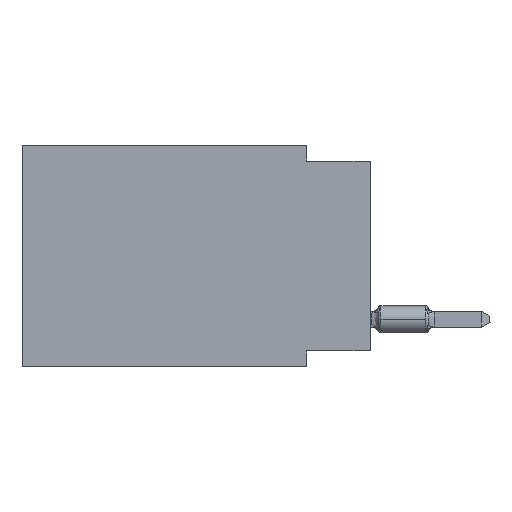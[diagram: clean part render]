
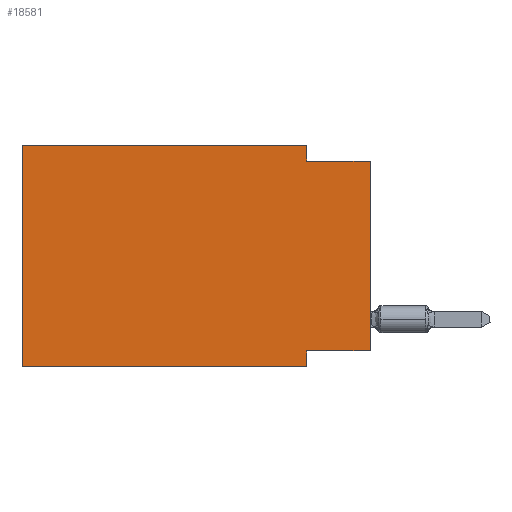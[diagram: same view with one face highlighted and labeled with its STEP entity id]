
A CAD part, left-side view. The second image highlights one B-rep face of the part: STEP entity #18581.
In plain terms, the highlighted planar face has unit normal (-1, 0, 0).
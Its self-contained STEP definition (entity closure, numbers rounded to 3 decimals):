
#150 = EDGE_CURVE ( 'NONE', #3956, #7314, #4441, .T. ) ;
#947 = ORIENTED_EDGE ( 'NONE', *, *, #33464, .F. ) ;
#1435 = DIRECTION ( 'NONE',  ( 0., 0., 1. ) ) ;
#3645 = DIRECTION ( 'NONE',  ( 0., -1., 0. ) ) ;
#3956 = VERTEX_POINT ( 'NONE', #19275 ) ;
#4171 = VERTEX_POINT ( 'NONE', #24043 ) ;
#4428 = ORIENTED_EDGE ( 'NONE', *, *, #22946, .F. ) ;
#4441 = LINE ( 'NONE', #12628, #32275 ) ;
#5887 = VECTOR ( 'NONE', #3645, 1000. ) ;
#6837 = ORIENTED_EDGE ( 'NONE', *, *, #17227, .F. ) ;
#7088 = FACE_OUTER_BOUND ( 'NONE', #22994, .T. ) ;
#7314 = VERTEX_POINT ( 'NONE', #27751 ) ;
#7979 = DIRECTION ( 'NONE',  ( 0., -1., 0. ) ) ;
#8051 = VECTOR ( 'NONE', #27856, 1000. ) ;
#9143 = CARTESIAN_POINT ( 'NONE',  ( 0., 0., -0.635 ) ) ;
#10374 = CARTESIAN_POINT ( 'NONE',  ( 0., 13.97, 0. ) ) ;
#10530 = ORIENTED_EDGE ( 'NONE', *, *, #19346, .F. ) ;
#10994 = VERTEX_POINT ( 'NONE', #25387 ) ;
#11420 = LINE ( 'NONE', #22230, #17637 ) ;
#11453 = VECTOR ( 'NONE', #1435, 1000. ) ;
#11707 = CARTESIAN_POINT ( 'NONE',  ( 0., 0., -8.255 ) ) ;
#11760 = CARTESIAN_POINT ( 'NONE',  ( 0., 13.97, 0. ) ) ;
#12628 = CARTESIAN_POINT ( 'NONE',  ( 0., 13.97, -8.89 ) ) ;
#13646 = VERTEX_POINT ( 'NONE', #28671 ) ;
#13700 = ORIENTED_EDGE ( 'NONE', *, *, #17064, .F. ) ;
#17064 = EDGE_CURVE ( 'NONE', #10994, #18953, #30346, .T. ) ;
#17227 = EDGE_CURVE ( 'NONE', #18953, #7314, #17358, .T. ) ;
#17240 = ORIENTED_EDGE ( 'NONE', *, *, #28916, .T. ) ;
#17358 = LINE ( 'NONE', #20036, #34678 ) ;
#17637 = VECTOR ( 'NONE', #27726, 1000. ) ;
#17889 = DIRECTION ( 'NONE',  ( 0., 0., -1. ) ) ;
#18253 = DIRECTION ( 'NONE',  ( 1., 0., 0. ) ) ;
#18581 = ADVANCED_FACE ( 'NONE', ( #7088 ), #23927, .F. ) ;
#18953 = VERTEX_POINT ( 'NONE', #22840 ) ;
#19275 = CARTESIAN_POINT ( 'NONE',  ( 0., 13.97, -8.89 ) ) ;
#19346 = EDGE_CURVE ( 'NONE', #20024, #4171, #19947, .T. ) ;
#19947 = LINE ( 'NONE', #9143, #5887 ) ;
#20024 = VERTEX_POINT ( 'NONE', #29822 ) ;
#20036 = CARTESIAN_POINT ( 'NONE',  ( 0., 2.54, -8.89 ) ) ;
#20688 = EDGE_CURVE ( 'NONE', #3956, #23898, #31848, .T. ) ;
#20732 = CARTESIAN_POINT ( 'NONE',  ( 0., 0., 0. ) ) ;
#21433 = LINE ( 'NONE', #32287, #28736 ) ;
#22230 = CARTESIAN_POINT ( 'NONE',  ( 0., 2.54, 0. ) ) ;
#22840 = CARTESIAN_POINT ( 'NONE',  ( 0., 2.54, -8.255 ) ) ;
#22946 = EDGE_CURVE ( 'NONE', #23898, #13646, #21433, .T. ) ;
#22994 = EDGE_LOOP ( 'NONE', ( #17240, #10530, #947, #4428, #24025, #33899, #6837, #13700 ) ) ;
#23898 = VERTEX_POINT ( 'NONE', #11760 ) ;
#23927 = PLANE ( 'NONE',  #30807 ) ;
#24025 = ORIENTED_EDGE ( 'NONE', *, *, #20688, .F. ) ;
#24043 = CARTESIAN_POINT ( 'NONE',  ( 0., 0., -0.635 ) ) ;
#24264 = VECTOR ( 'NONE', #29332, 1000. ) ;
#25387 = CARTESIAN_POINT ( 'NONE',  ( 0., 0., -8.255 ) ) ;
#26577 = CARTESIAN_POINT ( 'NONE',  ( 0., 13.97, 0. ) ) ;
#27726 = DIRECTION ( 'NONE',  ( 0., 0., -1. ) ) ;
#27751 = CARTESIAN_POINT ( 'NONE',  ( 0., 2.54, -8.89 ) ) ;
#27856 = DIRECTION ( 'NONE',  ( 0., 1., 0. ) ) ;
#28192 = DIRECTION ( 'NONE',  ( 0., 0., -1. ) ) ;
#28671 = CARTESIAN_POINT ( 'NONE',  ( 0., 2.54, 0. ) ) ;
#28736 = VECTOR ( 'NONE', #7979, 1000. ) ;
#28916 = EDGE_CURVE ( 'NONE', #10994, #4171, #33885, .T. ) ;
#29332 = DIRECTION ( 'NONE',  ( 0., 0., 1. ) ) ;
#29822 = CARTESIAN_POINT ( 'NONE',  ( 0., 2.54, -0.635 ) ) ;
#30346 = LINE ( 'NONE', #11707, #8051 ) ;
#30807 = AXIS2_PLACEMENT_3D ( 'NONE', #26577, #18253, #17889 ) ;
#31848 = LINE ( 'NONE', #10374, #24264 ) ;
#32275 = VECTOR ( 'NONE', #34286, 1000. ) ;
#32287 = CARTESIAN_POINT ( 'NONE',  ( 0., 13.97, 0. ) ) ;
#33464 = EDGE_CURVE ( 'NONE', #13646, #20024, #11420, .T. ) ;
#33885 = LINE ( 'NONE', #20732, #11453 ) ;
#33899 = ORIENTED_EDGE ( 'NONE', *, *, #150, .T. ) ;
#34286 = DIRECTION ( 'NONE',  ( 0., -1., 0. ) ) ;
#34678 = VECTOR ( 'NONE', #28192, 1000. ) ;
